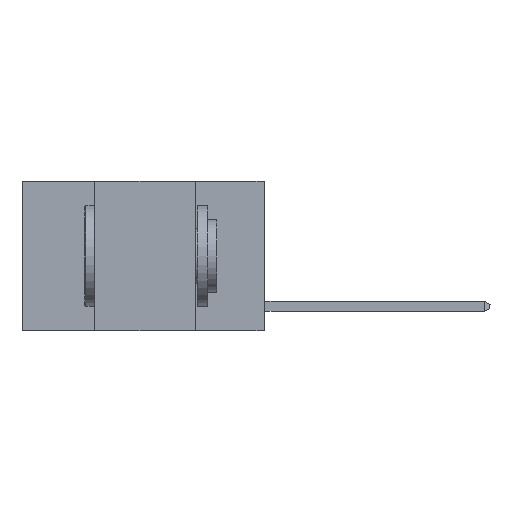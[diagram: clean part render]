
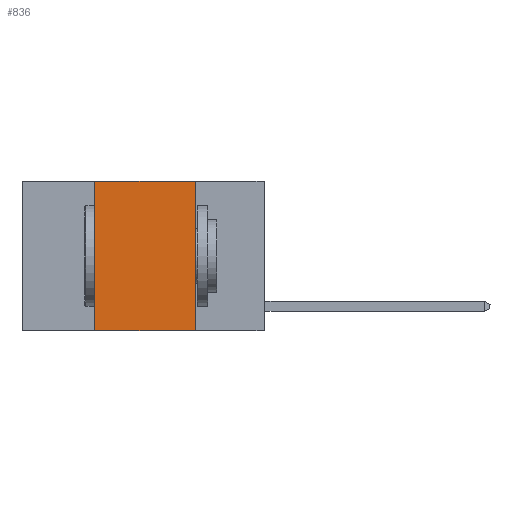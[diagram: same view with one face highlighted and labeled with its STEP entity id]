
A CAD part, left-side view. The second image highlights one B-rep face of the part: STEP entity #836.
In plain terms, the highlighted planar face has unit normal (-1, 0, 0).
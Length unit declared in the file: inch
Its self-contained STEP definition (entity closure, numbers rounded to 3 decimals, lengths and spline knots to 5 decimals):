
#294 = LINE ( 'NONE', #5449, #7220 ) ;
#836 = ADVANCED_FACE ( 'NONE', ( #6509 ), #9743, .F. ) ;
#1091 = EDGE_CURVE ( 'NONE', #2956, #2950, #4087, .T. ) ;
#1268 = CARTESIAN_POINT ( 'NONE',  ( 0., 0.17, 0. ) ) ;
#1339 = LINE ( 'NONE', #3844, #1935 ) ;
#1935 = VECTOR ( 'NONE', #8074, 39.37008 ) ;
#1953 = CARTESIAN_POINT ( 'NONE',  ( 0., 0.42, 0. ) ) ;
#2481 = VERTEX_POINT ( 'NONE', #1953 ) ;
#2763 = EDGE_CURVE ( 'NONE', #2481, #10801, #9189, .T. ) ;
#2950 = VERTEX_POINT ( 'NONE', #10483 ) ;
#2956 = VERTEX_POINT ( 'NONE', #8012 ) ;
#3399 = DIRECTION ( 'NONE',  ( 0., -1., 0. ) ) ;
#3844 = CARTESIAN_POINT ( 'NONE',  ( 0., 0.42, 0. ) ) ;
#4087 = LINE ( 'NONE', #10897, #6105 ) ;
#4785 = DIRECTION ( 'NONE',  ( 0., 0., -1. ) ) ;
#5449 = CARTESIAN_POINT ( 'NONE',  ( 0., 0.17, 0. ) ) ;
#6105 = VECTOR ( 'NONE', #3399, 39.37008 ) ;
#6509 = FACE_OUTER_BOUND ( 'NONE', #10826, .T. ) ;
#7220 = VECTOR ( 'NONE', #8781, 39.37008 ) ;
#7736 = EDGE_CURVE ( 'NONE', #10801, #2950, #294, .T. ) ;
#7758 = DIRECTION ( 'NONE',  ( 0., -1., 0. ) ) ;
#7858 = EDGE_CURVE ( 'NONE', #2956, #2481, #1339, .T. ) ;
#8012 = CARTESIAN_POINT ( 'NONE',  ( 0., 0.42, -0.37 ) ) ;
#8074 = DIRECTION ( 'NONE',  ( 0., 0., 1. ) ) ;
#8117 = CARTESIAN_POINT ( 'NONE',  ( 0., 0.6, 0. ) ) ;
#8341 = ORIENTED_EDGE ( 'NONE', *, *, #7736, .F. ) ;
#8352 = ORIENTED_EDGE ( 'NONE', *, *, #2763, .F. ) ;
#8617 = ORIENTED_EDGE ( 'NONE', *, *, #7858, .F. ) ;
#8634 = ORIENTED_EDGE ( 'NONE', *, *, #1091, .T. ) ;
#8674 = VECTOR ( 'NONE', #7758, 39.37008 ) ;
#8781 = DIRECTION ( 'NONE',  ( 0., 0., -1. ) ) ;
#9189 = LINE ( 'NONE', #9404, #8674 ) ;
#9404 = CARTESIAN_POINT ( 'NONE',  ( 0., 0.6, 0. ) ) ;
#9743 = PLANE ( 'NONE',  #10280 ) ;
#9804 = DIRECTION ( 'NONE',  ( 1., 0., 0. ) ) ;
#10280 = AXIS2_PLACEMENT_3D ( 'NONE', #8117, #9804, #4785 ) ;
#10483 = CARTESIAN_POINT ( 'NONE',  ( 0., 0.17, -0.37 ) ) ;
#10801 = VERTEX_POINT ( 'NONE', #1268 ) ;
#10826 = EDGE_LOOP ( 'NONE', ( #8341, #8352, #8617, #8634 ) ) ;
#10897 = CARTESIAN_POINT ( 'NONE',  ( 0., 0.6, -0.37 ) ) ;
